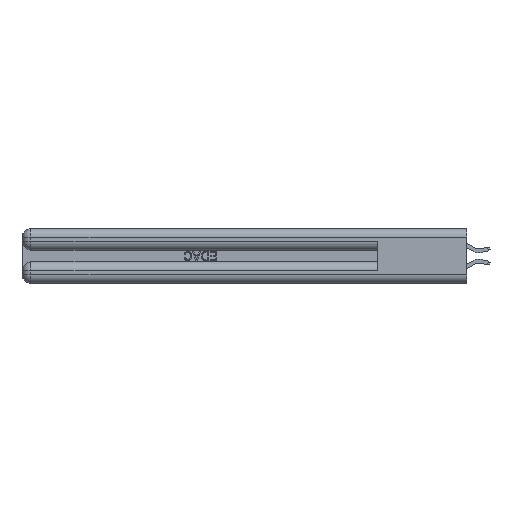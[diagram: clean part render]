
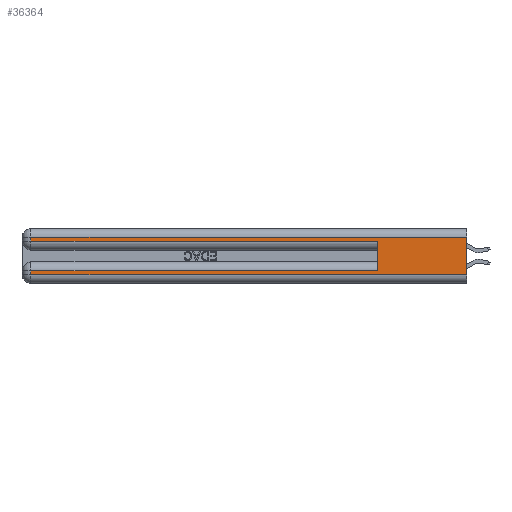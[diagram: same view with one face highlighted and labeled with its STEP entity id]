
A CAD part, left-side view. The second image highlights one B-rep face of the part: STEP entity #36364.
In plain terms, the highlighted planar face has unit normal (-1, 0, 0).
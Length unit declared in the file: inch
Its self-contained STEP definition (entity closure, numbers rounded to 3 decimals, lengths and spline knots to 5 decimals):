
#600 = VECTOR ( 'NONE', #35504, 39.37008 ) ;
#2339 = DIRECTION ( 'NONE',  ( 0., 1., 0. ) ) ;
#3219 = LINE ( 'NONE', #9671, #42280 ) ;
#3242 = EDGE_CURVE ( 'NONE', #39454, #21737, #4458, .T. ) ;
#3395 = CARTESIAN_POINT ( 'NONE',  ( 0., 0., 0.285 ) ) ;
#3489 = VECTOR ( 'NONE', #16119, 39.37008 ) ;
#4303 = CARTESIAN_POINT ( 'NONE',  ( 0., 2.94, 0.06 ) ) ;
#4330 = CARTESIAN_POINT ( 'NONE',  ( 0., 2.94, 0.37 ) ) ;
#4458 = LINE ( 'NONE', #23543, #26230 ) ;
#5192 = ORIENTED_EDGE ( 'NONE', *, *, #9807, .T. ) ;
#6498 = CARTESIAN_POINT ( 'NONE',  ( 0., 0., 0.06 ) ) ;
#6503 = LINE ( 'NONE', #14010, #36100 ) ;
#6785 = CARTESIAN_POINT ( 'NONE',  ( 0., 0., 0.31 ) ) ;
#7175 = DIRECTION ( 'NONE',  ( 1., 0., 0. ) ) ;
#8203 = VERTEX_POINT ( 'NONE', #30412 ) ;
#8233 = LINE ( 'NONE', #21029, #19965 ) ;
#8768 = CARTESIAN_POINT ( 'NONE',  ( 0., 0., 0.31 ) ) ;
#9671 = CARTESIAN_POINT ( 'NONE',  ( 0., 0., 0.37 ) ) ;
#9807 = EDGE_CURVE ( 'NONE', #21737, #15028, #10787, .T. ) ;
#10787 = LINE ( 'NONE', #4330, #15296 ) ;
#11368 = VERTEX_POINT ( 'NONE', #20656 ) ;
#14010 = CARTESIAN_POINT ( 'NONE',  ( 0., 2.94, 0.37 ) ) ;
#14321 = ORIENTED_EDGE ( 'NONE', *, *, #29112, .T. ) ;
#14612 = LINE ( 'NONE', #8768, #3489 ) ;
#15028 = VERTEX_POINT ( 'NONE', #4303 ) ;
#15296 = VECTOR ( 'NONE', #39768, 39.37008 ) ;
#15683 = LINE ( 'NONE', #3395, #600 ) ;
#16119 = DIRECTION ( 'NONE',  ( 0., 1., 0. ) ) ;
#17131 = DIRECTION ( 'NONE',  ( 0., -1., 0. ) ) ;
#18089 = DIRECTION ( 'NONE',  ( 0., 0., -1. ) ) ;
#18714 = EDGE_CURVE ( 'NONE', #39454, #8203, #34616, .T. ) ;
#19965 = VECTOR ( 'NONE', #17131, 39.37008 ) ;
#20389 = EDGE_CURVE ( 'NONE', #40697, #38904, #3219, .T. ) ;
#20656 = CARTESIAN_POINT ( 'NONE',  ( 0., 2.94, 0.31 ) ) ;
#20703 = ORIENTED_EDGE ( 'NONE', *, *, #44404, .T. ) ;
#21029 = CARTESIAN_POINT ( 'NONE',  ( 0., 0., 0.06 ) ) ;
#21166 = ORIENTED_EDGE ( 'NONE', *, *, #44172, .T. ) ;
#21737 = VERTEX_POINT ( 'NONE', #33366 ) ;
#23543 = CARTESIAN_POINT ( 'NONE',  ( 0., 0., 0.085 ) ) ;
#24214 = DIRECTION ( 'NONE',  ( 0., 0., -1. ) ) ;
#24527 = CARTESIAN_POINT ( 'NONE',  ( 0., 0.6, 0.145 ) ) ;
#24671 = DIRECTION ( 'NONE',  ( 0., 0., 1. ) ) ;
#24864 = CARTESIAN_POINT ( 'NONE',  ( 0., 2.94, 0.285 ) ) ;
#26230 = VECTOR ( 'NONE', #2339, 39.37008 ) ;
#27809 = CARTESIAN_POINT ( 'NONE',  ( 0., 0.6, 0.085 ) ) ;
#28141 = EDGE_CURVE ( 'NONE', #40697, #11368, #14612, .T. ) ;
#28708 = PLANE ( 'NONE',  #44994 ) ;
#29112 = EDGE_CURVE ( 'NONE', #33404, #8203, #15683, .T. ) ;
#29667 = ORIENTED_EDGE ( 'NONE', *, *, #20389, .F. ) ;
#30081 = ORIENTED_EDGE ( 'NONE', *, *, #28141, .T. ) ;
#30412 = CARTESIAN_POINT ( 'NONE',  ( 0., 0.6, 0.285 ) ) ;
#30957 = ORIENTED_EDGE ( 'NONE', *, *, #18714, .F. ) ;
#32106 = DIRECTION ( 'NONE',  ( 0., 0., -1. ) ) ;
#33366 = CARTESIAN_POINT ( 'NONE',  ( 0., 2.94, 0.085 ) ) ;
#33404 = VERTEX_POINT ( 'NONE', #24864 ) ;
#34616 = LINE ( 'NONE', #24527, #42994 ) ;
#34705 = ORIENTED_EDGE ( 'NONE', *, *, #3242, .T. ) ;
#35040 = FACE_OUTER_BOUND ( 'NONE', #36277, .T. ) ;
#35504 = DIRECTION ( 'NONE',  ( 0., -1., 0. ) ) ;
#36100 = VECTOR ( 'NONE', #32106, 39.37008 ) ;
#36277 = EDGE_LOOP ( 'NONE', ( #29667, #30081, #20703, #14321, #30957, #34705, #5192, #21166 ) ) ;
#36364 = ADVANCED_FACE ( 'NONE', ( #35040 ), #28708, .F. ) ;
#38904 = VERTEX_POINT ( 'NONE', #6498 ) ;
#39454 = VERTEX_POINT ( 'NONE', #27809 ) ;
#39768 = DIRECTION ( 'NONE',  ( 0., 0., -1. ) ) ;
#40697 = VERTEX_POINT ( 'NONE', #6785 ) ;
#42280 = VECTOR ( 'NONE', #24214, 39.37008 ) ;
#42994 = VECTOR ( 'NONE', #24671, 39.37008 ) ;
#43054 = CARTESIAN_POINT ( 'NONE',  ( 0., 0., 0.37 ) ) ;
#44172 = EDGE_CURVE ( 'NONE', #15028, #38904, #8233, .T. ) ;
#44404 = EDGE_CURVE ( 'NONE', #11368, #33404, #6503, .T. ) ;
#44994 = AXIS2_PLACEMENT_3D ( 'NONE', #43054, #7175, #18089 ) ;
